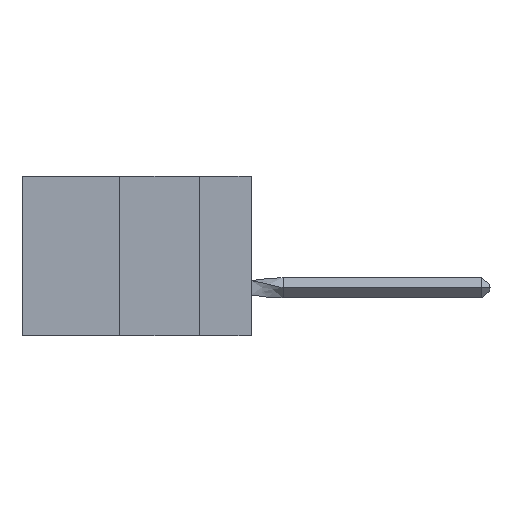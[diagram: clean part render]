
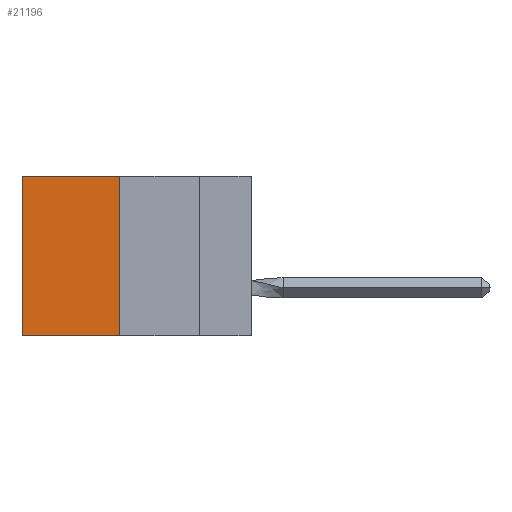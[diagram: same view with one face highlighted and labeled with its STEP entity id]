
A CAD part, left-side view. The second image highlights one B-rep face of the part: STEP entity #21196.
In plain terms, the highlighted planar face has unit normal (-1, 0, 0).
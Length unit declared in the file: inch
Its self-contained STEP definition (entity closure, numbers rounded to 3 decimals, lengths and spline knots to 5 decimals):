
#91 = VECTOR ( 'NONE', #11614, 39.37008 ) ;
#189 = VERTEX_POINT ( 'NONE', #7007 ) ;
#649 = AXIS2_PLACEMENT_3D ( 'NONE', #20440, #13399, #9746 ) ;
#1142 = ORIENTED_EDGE ( 'NONE', *, *, #13823, .T. ) ;
#1482 = ORIENTED_EDGE ( 'NONE', *, *, #2798, .F. ) ;
#2798 = EDGE_CURVE ( 'NONE', #9978, #189, #10507, .T. ) ;
#3553 = CARTESIAN_POINT ( 'NONE',  ( 0.305, 0.413, 0. ) ) ;
#4090 = VERTEX_POINT ( 'NONE', #18064 ) ;
#4264 = EDGE_CURVE ( 'NONE', #10039, #9978, #13450, .T. ) ;
#4529 = ORIENTED_EDGE ( 'NONE', *, *, #4264, .F. ) ;
#5069 = EDGE_LOOP ( 'NONE', ( #21684, #1482, #4529, #1142 ) ) ;
#5242 = CARTESIAN_POINT ( 'NONE',  ( 0.305, 0.413, -0.5 ) ) ;
#6113 = CARTESIAN_POINT ( 'NONE',  ( 0.305, 0.72, -0.5 ) ) ;
#7007 = CARTESIAN_POINT ( 'NONE',  ( 0.305, 0.72, -0.5 ) ) ;
#9036 = EDGE_CURVE ( 'NONE', #4090, #189, #15319, .T. ) ;
#9746 = DIRECTION ( 'NONE',  ( 0., 0., -1. ) ) ;
#9964 = VECTOR ( 'NONE', #17455, 39.37008 ) ;
#9978 = VERTEX_POINT ( 'NONE', #20878 ) ;
#10039 = VERTEX_POINT ( 'NONE', #11942 ) ;
#10374 = DIRECTION ( 'NONE',  ( 0., 1., 0. ) ) ;
#10507 = LINE ( 'NONE', #5242, #9964 ) ;
#11614 = DIRECTION ( 'NONE',  ( 0., 0., -1. ) ) ;
#11942 = CARTESIAN_POINT ( 'NONE',  ( 0.305, 0.413, 0. ) ) ;
#12561 = VECTOR ( 'NONE', #18330, 39.37008 ) ;
#13399 = DIRECTION ( 'NONE',  ( 1., 0., 0. ) ) ;
#13450 = LINE ( 'NONE', #20488, #91 ) ;
#13823 = EDGE_CURVE ( 'NONE', #10039, #4090, #14279, .T. ) ;
#14279 = LINE ( 'NONE', #3553, #16483 ) ;
#15309 = FACE_OUTER_BOUND ( 'NONE', #5069, .T. ) ;
#15319 = LINE ( 'NONE', #6113, #12561 ) ;
#16483 = VECTOR ( 'NONE', #10374, 39.37008 ) ;
#17455 = DIRECTION ( 'NONE',  ( 0., 1., 0. ) ) ;
#18064 = CARTESIAN_POINT ( 'NONE',  ( 0.305, 0.72, 0. ) ) ;
#18330 = DIRECTION ( 'NONE',  ( 0., 0., -1. ) ) ;
#20286 = PLANE ( 'NONE',  #649 ) ;
#20440 = CARTESIAN_POINT ( 'NONE',  ( 0.305, 0.413, -0.5 ) ) ;
#20488 = CARTESIAN_POINT ( 'NONE',  ( 0.305, 0.413, -0.5 ) ) ;
#20878 = CARTESIAN_POINT ( 'NONE',  ( 0.305, 0.413, -0.5 ) ) ;
#21196 = ADVANCED_FACE ( 'NONE', ( #15309 ), #20286, .F. ) ;
#21684 = ORIENTED_EDGE ( 'NONE', *, *, #9036, .T. ) ;
